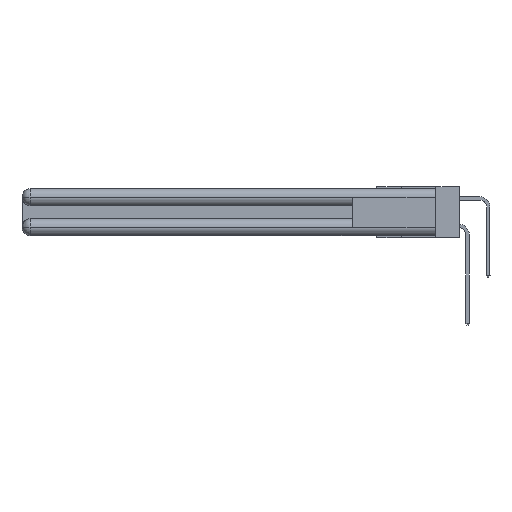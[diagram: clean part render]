
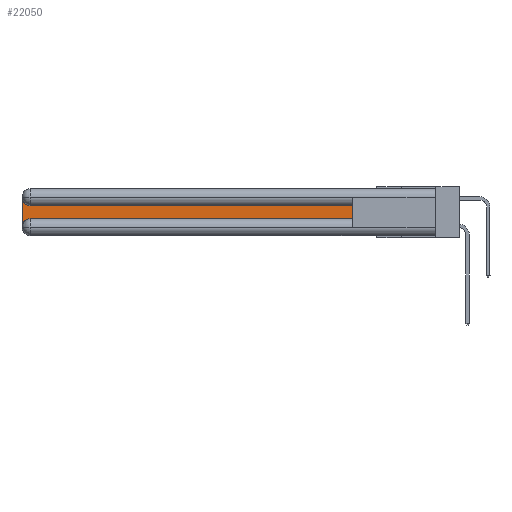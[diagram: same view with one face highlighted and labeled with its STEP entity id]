
A CAD part, left-side view. The second image highlights one B-rep face of the part: STEP entity #22050.
In plain terms, the highlighted planar face has unit normal (-1, 0, 0).
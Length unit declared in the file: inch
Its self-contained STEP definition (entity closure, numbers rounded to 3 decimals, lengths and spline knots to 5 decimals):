
#269 = ORIENTED_EDGE ( 'NONE', *, *, #18229, .T. ) ;
#1384 = VERTEX_POINT ( 'NONE', #13189 ) ;
#1544 = EDGE_CURVE ( 'NONE', #19234, #3842, #5015, .T. ) ;
#2364 = DIRECTION ( 'NONE',  ( 1., 0., 0. ) ) ;
#3842 = VERTEX_POINT ( 'NONE', #6950 ) ;
#5015 = LINE ( 'NONE', #22518, #33700 ) ;
#5777 = LINE ( 'NONE', #31664, #17692 ) ;
#5867 = EDGE_CURVE ( 'NONE', #3842, #15716, #30593, .T. ) ;
#6950 = CARTESIAN_POINT ( 'NONE',  ( 0.075, 0.6, -0.1225 ) ) ;
#7385 = EDGE_CURVE ( 'NONE', #18232, #1384, #5777, .T. ) ;
#8545 = CARTESIAN_POINT ( 'NONE',  ( 0.075, 0.6, -0.1225 ) ) ;
#9043 = CIRCLE ( 'NONE', #13076, 0.06 ) ;
#10848 = DIRECTION ( 'NONE',  ( 0., 0., 1. ) ) ;
#12415 = CARTESIAN_POINT ( 'NONE',  ( 0.075, 2.94, -0.2175 ) ) ;
#13076 = AXIS2_PLACEMENT_3D ( 'NONE', #23998, #19006, #33028 ) ;
#13189 = CARTESIAN_POINT ( 'NONE',  ( 0.075, 3., -0.2775 ) ) ;
#14472 = LINE ( 'NONE', #26212, #31342 ) ;
#15716 = VERTEX_POINT ( 'NONE', #24572 ) ;
#16130 = DIRECTION ( 'NONE',  ( 0., 0., -1. ) ) ;
#16529 = ORIENTED_EDGE ( 'NONE', *, *, #30937, .T. ) ;
#16639 = EDGE_LOOP ( 'NONE', ( #23410, #269, #29906, #27437, #16529, #18962 ) ) ;
#16703 = AXIS2_PLACEMENT_3D ( 'NONE', #19396, #25327, #22272 ) ;
#17018 = DIRECTION ( 'NONE',  ( 0., 1., 0. ) ) ;
#17692 = VECTOR ( 'NONE', #26155, 39.37008 ) ;
#18229 = EDGE_CURVE ( 'NONE', #15716, #18232, #28669, .T. ) ;
#18232 = VERTEX_POINT ( 'NONE', #36364 ) ;
#18962 = ORIENTED_EDGE ( 'NONE', *, *, #1544, .T. ) ;
#19006 = DIRECTION ( 'NONE',  ( 1., 0., 0. ) ) ;
#19234 = VERTEX_POINT ( 'NONE', #21507 ) ;
#19396 = CARTESIAN_POINT ( 'NONE',  ( 0.075, 2.94, -0.0625 ) ) ;
#19527 = PLANE ( 'NONE',  #30974 ) ;
#21507 = CARTESIAN_POINT ( 'NONE',  ( 0.075, 0.6, -0.2175 ) ) ;
#21837 = FACE_OUTER_BOUND ( 'NONE', #16639, .T. ) ;
#22050 = ADVANCED_FACE ( 'NONE', ( #21837 ), #19527, .F. ) ;
#22272 = DIRECTION ( 'NONE',  ( 0., 0., -1. ) ) ;
#22280 = VECTOR ( 'NONE', #17018, 39.37008 ) ;
#22518 = CARTESIAN_POINT ( 'NONE',  ( 0.075, 0.6, -0.2175 ) ) ;
#23410 = ORIENTED_EDGE ( 'NONE', *, *, #5867, .T. ) ;
#23998 = CARTESIAN_POINT ( 'NONE',  ( 0.075, 2.94, -0.2775 ) ) ;
#24572 = CARTESIAN_POINT ( 'NONE',  ( 0.075, 2.94, -0.1225 ) ) ;
#25327 = DIRECTION ( 'NONE',  ( 1., 0., 0. ) ) ;
#26155 = DIRECTION ( 'NONE',  ( 0., 0., -1. ) ) ;
#26212 = CARTESIAN_POINT ( 'NONE',  ( 0.075, 0.6, -0.2175 ) ) ;
#27437 = ORIENTED_EDGE ( 'NONE', *, *, #33590, .T. ) ;
#28187 = VERTEX_POINT ( 'NONE', #12415 ) ;
#28669 = CIRCLE ( 'NONE', #16703, 0.06 ) ;
#29906 = ORIENTED_EDGE ( 'NONE', *, *, #7385, .T. ) ;
#30593 = LINE ( 'NONE', #8545, #22280 ) ;
#30842 = CARTESIAN_POINT ( 'NONE',  ( 0.075, 3., -0.1225 ) ) ;
#30937 = EDGE_CURVE ( 'NONE', #28187, #19234, #14472, .T. ) ;
#30974 = AXIS2_PLACEMENT_3D ( 'NONE', #30842, #2364, #16130 ) ;
#31342 = VECTOR ( 'NONE', #34561, 39.37008 ) ;
#31664 = CARTESIAN_POINT ( 'NONE',  ( 0.075, 3., -0.2175 ) ) ;
#33028 = DIRECTION ( 'NONE',  ( 0., 0., -1. ) ) ;
#33590 = EDGE_CURVE ( 'NONE', #1384, #28187, #9043, .T. ) ;
#33700 = VECTOR ( 'NONE', #10848, 39.37008 ) ;
#34561 = DIRECTION ( 'NONE',  ( 0., -1., 0. ) ) ;
#36364 = CARTESIAN_POINT ( 'NONE',  ( 0.075, 3., -0.0625 ) ) ;
